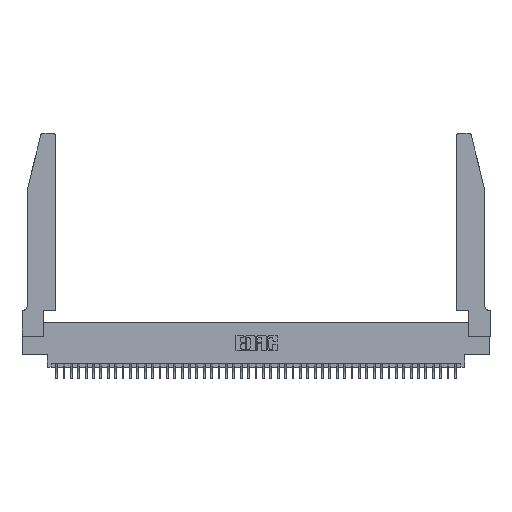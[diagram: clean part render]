
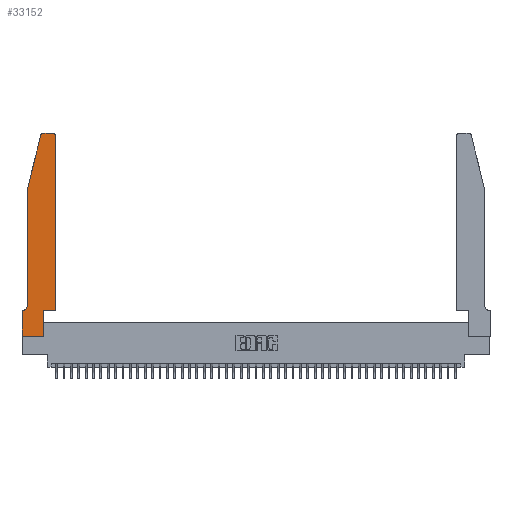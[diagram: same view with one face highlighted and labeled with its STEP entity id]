
A CAD part, top view. The second image highlights one B-rep face of the part: STEP entity #33152.
In plain terms, the highlighted planar face has unit normal (0, 0, 1).
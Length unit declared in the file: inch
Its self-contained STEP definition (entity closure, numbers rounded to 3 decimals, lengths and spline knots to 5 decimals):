
#294 = CARTESIAN_POINT ( 'NONE',  ( 0., 0., 0.37 ) ) ;
#1430 = VECTOR ( 'NONE', #21513, 39.37008 ) ;
#1722 = CARTESIAN_POINT ( 'NONE',  ( 0.284, 2.72, 0.37 ) ) ;
#2312 = DIRECTION ( 'NONE',  ( -1., 0., 0. ) ) ;
#3378 = CARTESIAN_POINT ( 'NONE',  ( 0., 0., 0.37 ) ) ;
#4698 = EDGE_CURVE ( 'NONE', #39887, #17928, #40316, .T. ) ;
#5078 = DIRECTION ( 'NONE',  ( -1., 0., 0. ) ) ;
#5559 = CARTESIAN_POINT ( 'NONE',  ( 0.0055, 0.42, 0.37 ) ) ;
#5747 = CARTESIAN_POINT ( 'NONE',  ( 0.0755, 2., 0.37 ) ) ;
#5790 = ORIENTED_EDGE ( 'NONE', *, *, #34923, .T. ) ;
#6495 = EDGE_CURVE ( 'NONE', #34190, #30076, #12613, .T. ) ;
#7581 = VERTEX_POINT ( 'NONE', #9078 ) ;
#7892 = VECTOR ( 'NONE', #5078, 39.37008 ) ;
#8794 = VECTOR ( 'NONE', #2312, 39.37008 ) ;
#9078 = CARTESIAN_POINT ( 'NONE',  ( 0.284, 2.75, 0.37 ) ) ;
#10365 = DIRECTION ( 'NONE',  ( 1., 0., 0. ) ) ;
#11419 = DIRECTION ( 'NONE',  ( 1., 0., 0. ) ) ;
#11831 = ORIENTED_EDGE ( 'NONE', *, *, #4698, .T. ) ;
#12508 = CIRCLE ( 'NONE', #14715, 0.03 ) ;
#12613 = LINE ( 'NONE', #294, #29462 ) ;
#12818 = DIRECTION ( 'NONE',  ( 0., -1., 0. ) ) ;
#12980 = ORIENTED_EDGE ( 'NONE', *, *, #16127, .T. ) ;
#13772 = EDGE_LOOP ( 'NONE', ( #46132, #21593, #11831, #17437, #12980, #35016, #36723, #5790, #34349, #44946, #37848, #45828 ) ) ;
#14715 = AXIS2_PLACEMENT_3D ( 'NONE', #1722, #23349, #42083 ) ;
#14963 = LINE ( 'NONE', #18841, #8794 ) ;
#15137 = DIRECTION ( 'NONE',  ( 0., 1., 0. ) ) ;
#16127 = EDGE_CURVE ( 'NONE', #25276, #28991, #23716, .T. ) ;
#16603 = EDGE_CURVE ( 'NONE', #7581, #39887, #12508, .T. ) ;
#16922 = LINE ( 'NONE', #43737, #18043 ) ;
#17395 = AXIS2_PLACEMENT_3D ( 'NONE', #45384, #38112, #27450 ) ;
#17437 = ORIENTED_EDGE ( 'NONE', *, *, #24694, .T. ) ;
#17491 = EDGE_CURVE ( 'NONE', #32147, #35211, #16922, .T. ) ;
#17501 = EDGE_CURVE ( 'NONE', #28991, #34190, #37695, .T. ) ;
#17928 = VERTEX_POINT ( 'NONE', #5747 ) ;
#18027 = CARTESIAN_POINT ( 'NONE',  ( 0.0755, 0.42, 0.37 ) ) ;
#18043 = VECTOR ( 'NONE', #15137, 39.37008 ) ;
#18841 = CARTESIAN_POINT ( 'NONE',  ( 0.2605, 2.75, 0.37 ) ) ;
#19551 = DIRECTION ( 'NONE',  ( 0., 0., -1. ) ) ;
#19892 = EDGE_CURVE ( 'NONE', #21516, #7581, #14963, .T. ) ;
#21251 = DIRECTION ( 'NONE',  ( 1., 0., 0. ) ) ;
#21273 = EDGE_CURVE ( 'NONE', #35211, #33456, #45793, .T. ) ;
#21344 = CARTESIAN_POINT ( 'NONE',  ( 0.0055, 0.35, 0.37 ) ) ;
#21513 = DIRECTION ( 'NONE',  ( 0., 1., 0. ) ) ;
#21516 = VERTEX_POINT ( 'NONE', #41450 ) ;
#21593 = ORIENTED_EDGE ( 'NONE', *, *, #16603, .T. ) ;
#21668 = EDGE_CURVE ( 'NONE', #33456, #45482, #43562, .T. ) ;
#21944 = LINE ( 'NONE', #43545, #43886 ) ;
#22144 = DIRECTION ( 'NONE',  ( 0., -1., 0. ) ) ;
#22797 = CARTESIAN_POINT ( 'NONE',  ( 0.25487, 2.72718, 0.37 ) ) ;
#22856 = CIRCLE ( 'NONE', #17395, 0.03 ) ;
#23349 = DIRECTION ( 'NONE',  ( 0., 0., 1. ) ) ;
#23716 = CIRCLE ( 'NONE', #37280, 0.07 ) ;
#24352 = DIRECTION ( 'NONE',  ( 0., 0., 1. ) ) ;
#24694 = EDGE_CURVE ( 'NONE', #17928, #25276, #21944, .T. ) ;
#25276 = VERTEX_POINT ( 'NONE', #18027 ) ;
#25712 = VECTOR ( 'NONE', #38333, 39.37008 ) ;
#26820 = AXIS2_PLACEMENT_3D ( 'NONE', #42592, #24352, #10365 ) ;
#27450 = DIRECTION ( 'NONE',  ( 1., 0., 0. ) ) ;
#28261 = VECTOR ( 'NONE', #11419, 39.37008 ) ;
#28991 = VERTEX_POINT ( 'NONE', #21344 ) ;
#29462 = VECTOR ( 'NONE', #12818, 39.37008 ) ;
#30076 = VERTEX_POINT ( 'NONE', #30374 ) ;
#30374 = CARTESIAN_POINT ( 'NONE',  ( 0., 0., 0.37 ) ) ;
#30883 = FACE_OUTER_BOUND ( 'NONE', #13772, .T. ) ;
#31682 = CARTESIAN_POINT ( 'NONE',  ( 0., 0.35, 0.37 ) ) ;
#32147 = VERTEX_POINT ( 'NONE', #39529 ) ;
#33152 = ADVANCED_FACE ( 'NONE', ( #30883 ), #46072, .T. ) ;
#33456 = VERTEX_POINT ( 'NONE', #39872 ) ;
#33788 = CARTESIAN_POINT ( 'NONE',  ( 0.0755, 0.35, 0.37 ) ) ;
#34190 = VERTEX_POINT ( 'NONE', #31682 ) ;
#34349 = ORIENTED_EDGE ( 'NONE', *, *, #17491, .T. ) ;
#34731 = CARTESIAN_POINT ( 'NONE',  ( 0.4505, 2.72, 0.37 ) ) ;
#34923 = EDGE_CURVE ( 'NONE', #30076, #32147, #42692, .T. ) ;
#35016 = ORIENTED_EDGE ( 'NONE', *, *, #17501, .T. ) ;
#35211 = VERTEX_POINT ( 'NONE', #43873 ) ;
#35892 = EDGE_CURVE ( 'NONE', #45482, #21516, #22856, .T. ) ;
#36384 = CARTESIAN_POINT ( 'NONE',  ( 0.4505, 0.35, 0.37 ) ) ;
#36723 = ORIENTED_EDGE ( 'NONE', *, *, #6495, .T. ) ;
#37280 = AXIS2_PLACEMENT_3D ( 'NONE', #5559, #19551, #41415 ) ;
#37695 = LINE ( 'NONE', #33788, #7892 ) ;
#37848 = ORIENTED_EDGE ( 'NONE', *, *, #21668, .T. ) ;
#38112 = DIRECTION ( 'NONE',  ( 0., 0., 1. ) ) ;
#38333 = DIRECTION ( 'NONE',  ( -0.239, -0.971, 0. ) ) ;
#39397 = CARTESIAN_POINT ( 'NONE',  ( 0.4505, 0.35, 0.37 ) ) ;
#39529 = CARTESIAN_POINT ( 'NONE',  ( 0.2865, 0., 0.37 ) ) ;
#39872 = CARTESIAN_POINT ( 'NONE',  ( 0.4505, 0.35, 0.37 ) ) ;
#39887 = VERTEX_POINT ( 'NONE', #22797 ) ;
#40316 = LINE ( 'NONE', #41492, #25712 ) ;
#41415 = DIRECTION ( 'NONE',  ( -1., 0., 0. ) ) ;
#41450 = CARTESIAN_POINT ( 'NONE',  ( 0.4205, 2.75, 0.37 ) ) ;
#41492 = CARTESIAN_POINT ( 'NONE',  ( 0.0755, 2., 0.37 ) ) ;
#41563 = VECTOR ( 'NONE', #21251, 39.37008 ) ;
#42083 = DIRECTION ( 'NONE',  ( 1., 0., 0. ) ) ;
#42592 = CARTESIAN_POINT ( 'NONE',  ( 0., 0.35, 0.37 ) ) ;
#42692 = LINE ( 'NONE', #3378, #41563 ) ;
#43545 = CARTESIAN_POINT ( 'NONE',  ( 0.0755, 2., 0.37 ) ) ;
#43562 = LINE ( 'NONE', #36384, #1430 ) ;
#43737 = CARTESIAN_POINT ( 'NONE',  ( 0.2865, 0.35, 0.37 ) ) ;
#43873 = CARTESIAN_POINT ( 'NONE',  ( 0.2865, 0.35, 0.37 ) ) ;
#43886 = VECTOR ( 'NONE', #22144, 39.37008 ) ;
#44946 = ORIENTED_EDGE ( 'NONE', *, *, #21273, .T. ) ;
#45384 = CARTESIAN_POINT ( 'NONE',  ( 0.4205, 2.72, 0.37 ) ) ;
#45482 = VERTEX_POINT ( 'NONE', #34731 ) ;
#45793 = LINE ( 'NONE', #39397, #28261 ) ;
#45828 = ORIENTED_EDGE ( 'NONE', *, *, #35892, .T. ) ;
#46072 = PLANE ( 'NONE',  #26820 ) ;
#46132 = ORIENTED_EDGE ( 'NONE', *, *, #19892, .T. ) ;
